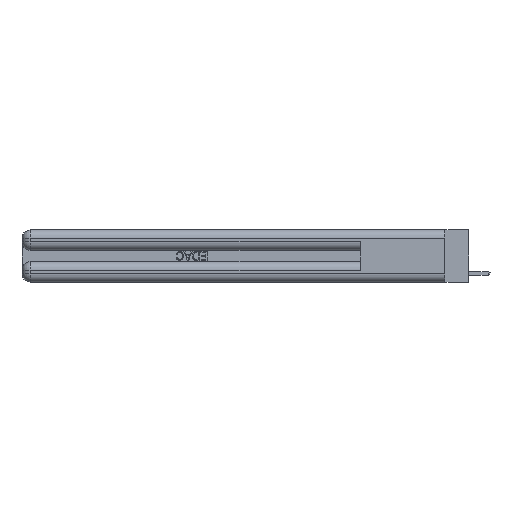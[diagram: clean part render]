
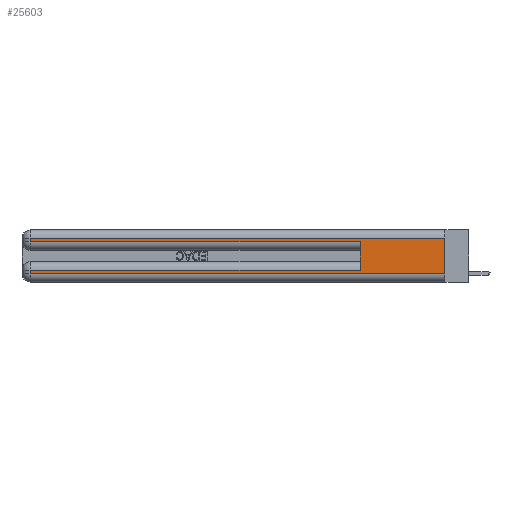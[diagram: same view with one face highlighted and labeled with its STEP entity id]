
A CAD part, left-side view. The second image highlights one B-rep face of the part: STEP entity #25603.
In plain terms, the highlighted planar face has unit normal (-1, 0, 0).
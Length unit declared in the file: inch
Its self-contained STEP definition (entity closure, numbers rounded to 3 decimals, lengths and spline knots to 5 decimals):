
#314 = VERTEX_POINT ( 'NONE', #3257 ) ;
#595 = LINE ( 'NONE', #19712, #12539 ) ;
#749 = VECTOR ( 'NONE', #14050, 39.37008 ) ;
#1351 = CARTESIAN_POINT ( 'NONE',  ( 0., 0.6, 0.285 ) ) ;
#1358 = EDGE_CURVE ( 'NONE', #1777, #8613, #7493, .T. ) ;
#1369 = VECTOR ( 'NONE', #5159, 39.37008 ) ;
#1469 = LINE ( 'NONE', #15779, #749 ) ;
#1682 = DIRECTION ( 'NONE',  ( 0., 0., -1. ) ) ;
#1777 = VERTEX_POINT ( 'NONE', #10407 ) ;
#2574 = EDGE_CURVE ( 'NONE', #314, #29100, #1469, .T. ) ;
#2662 = CARTESIAN_POINT ( 'NONE',  ( 0., 0.6, 0.145 ) ) ;
#3257 = CARTESIAN_POINT ( 'NONE',  ( 0., 2.94, 0.06 ) ) ;
#3756 = VECTOR ( 'NONE', #18532, 39.37008 ) ;
#4005 = CARTESIAN_POINT ( 'NONE',  ( 0., 2.94, 0.37 ) ) ;
#4660 = EDGE_CURVE ( 'NONE', #28536, #7304, #9627, .T. ) ;
#5159 = DIRECTION ( 'NONE',  ( 0., 1., 0. ) ) ;
#5354 = PLANE ( 'NONE',  #28876 ) ;
#5988 = CARTESIAN_POINT ( 'NONE',  ( 0., 2.94, 0.285 ) ) ;
#6876 = LINE ( 'NONE', #15078, #25249 ) ;
#7304 = VERTEX_POINT ( 'NONE', #1351 ) ;
#7339 = CARTESIAN_POINT ( 'NONE',  ( 0., 2.94, 0.31 ) ) ;
#7453 = CARTESIAN_POINT ( 'NONE',  ( 0., 0., 0.37 ) ) ;
#7493 = LINE ( 'NONE', #18695, #1369 ) ;
#7775 = FACE_OUTER_BOUND ( 'NONE', #15067, .T. ) ;
#8058 = ORIENTED_EDGE ( 'NONE', *, *, #22202, .T. ) ;
#8111 = ORIENTED_EDGE ( 'NONE', *, *, #2574, .T. ) ;
#8345 = LINE ( 'NONE', #4005, #24556 ) ;
#8613 = VERTEX_POINT ( 'NONE', #7339 ) ;
#8943 = EDGE_CURVE ( 'NONE', #26496, #314, #8345, .T. ) ;
#9053 = CARTESIAN_POINT ( 'NONE',  ( 0., 0., 0.37 ) ) ;
#9627 = LINE ( 'NONE', #2662, #17240 ) ;
#9905 = LINE ( 'NONE', #9053, #3756 ) ;
#10407 = CARTESIAN_POINT ( 'NONE',  ( 0., 0., 0.31 ) ) ;
#11433 = ORIENTED_EDGE ( 'NONE', *, *, #18860, .T. ) ;
#11877 = EDGE_CURVE ( 'NONE', #28536, #26496, #595, .T. ) ;
#11959 = LINE ( 'NONE', #28496, #15593 ) ;
#12539 = VECTOR ( 'NONE', #17399, 39.37008 ) ;
#14050 = DIRECTION ( 'NONE',  ( 0., -1., 0. ) ) ;
#15067 = EDGE_LOOP ( 'NONE', ( #18297, #29777, #11433, #8058, #28665, #29938, #28326, #8111 ) ) ;
#15078 = CARTESIAN_POINT ( 'NONE',  ( 0., 2.94, 0.37 ) ) ;
#15593 = VECTOR ( 'NONE', #24697, 39.37008 ) ;
#15779 = CARTESIAN_POINT ( 'NONE',  ( 0., 0., 0.06 ) ) ;
#16764 = DIRECTION ( 'NONE',  ( 1., 0., 0. ) ) ;
#17038 = DIRECTION ( 'NONE',  ( 0., 0., 1. ) ) ;
#17240 = VECTOR ( 'NONE', #17038, 39.37008 ) ;
#17399 = DIRECTION ( 'NONE',  ( 0., 1., 0. ) ) ;
#18297 = ORIENTED_EDGE ( 'NONE', *, *, #28450, .F. ) ;
#18532 = DIRECTION ( 'NONE',  ( 0., 0., -1. ) ) ;
#18695 = CARTESIAN_POINT ( 'NONE',  ( 0., 0., 0.31 ) ) ;
#18860 = EDGE_CURVE ( 'NONE', #8613, #22234, #6876, .T. ) ;
#19712 = CARTESIAN_POINT ( 'NONE',  ( 0., 0., 0.085 ) ) ;
#21343 = CARTESIAN_POINT ( 'NONE',  ( 0., 0., 0.06 ) ) ;
#22150 = CARTESIAN_POINT ( 'NONE',  ( 0., 2.94, 0.085 ) ) ;
#22202 = EDGE_CURVE ( 'NONE', #22234, #7304, #11959, .T. ) ;
#22234 = VERTEX_POINT ( 'NONE', #5988 ) ;
#24519 = DIRECTION ( 'NONE',  ( 0., 0., -1. ) ) ;
#24556 = VECTOR ( 'NONE', #1682, 39.37008 ) ;
#24697 = DIRECTION ( 'NONE',  ( 0., -1., 0. ) ) ;
#25249 = VECTOR ( 'NONE', #24519, 39.37008 ) ;
#25603 = ADVANCED_FACE ( 'NONE', ( #7775 ), #5354, .F. ) ;
#25970 = CARTESIAN_POINT ( 'NONE',  ( 0., 0.6, 0.085 ) ) ;
#26496 = VERTEX_POINT ( 'NONE', #22150 ) ;
#28251 = DIRECTION ( 'NONE',  ( 0., 0., -1. ) ) ;
#28326 = ORIENTED_EDGE ( 'NONE', *, *, #8943, .T. ) ;
#28450 = EDGE_CURVE ( 'NONE', #1777, #29100, #9905, .T. ) ;
#28496 = CARTESIAN_POINT ( 'NONE',  ( 0., 0., 0.285 ) ) ;
#28536 = VERTEX_POINT ( 'NONE', #25970 ) ;
#28665 = ORIENTED_EDGE ( 'NONE', *, *, #4660, .F. ) ;
#28876 = AXIS2_PLACEMENT_3D ( 'NONE', #7453, #16764, #28251 ) ;
#29100 = VERTEX_POINT ( 'NONE', #21343 ) ;
#29777 = ORIENTED_EDGE ( 'NONE', *, *, #1358, .T. ) ;
#29938 = ORIENTED_EDGE ( 'NONE', *, *, #11877, .T. ) ;
